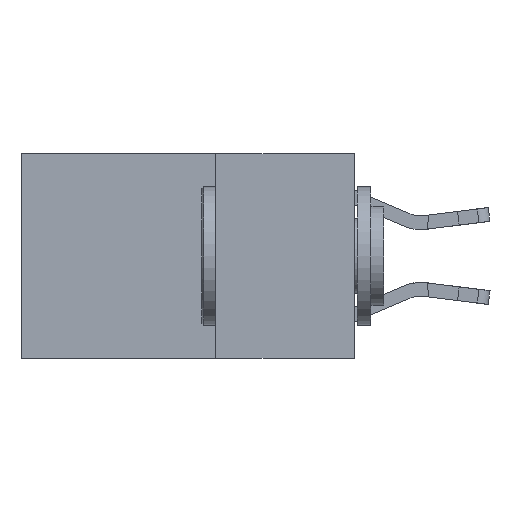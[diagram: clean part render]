
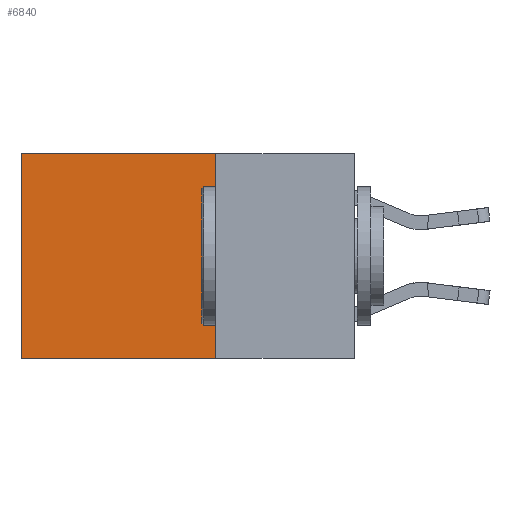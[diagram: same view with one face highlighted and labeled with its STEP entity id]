
A CAD part, left-side view. The second image highlights one B-rep face of the part: STEP entity #6840.
In plain terms, the highlighted planar face has unit normal (-1, 0, 0).
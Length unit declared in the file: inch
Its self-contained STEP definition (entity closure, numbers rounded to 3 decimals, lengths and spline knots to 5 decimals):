
#221 = EDGE_CURVE ( 'NONE', #16723, #18748, #11896, .T. ) ;
#668 = VERTEX_POINT ( 'NONE', #5026 ) ;
#800 = ORIENTED_EDGE ( 'NONE', *, *, #17229, .F. ) ;
#1386 = EDGE_CURVE ( 'NONE', #20524, #16723, #6756, .T. ) ;
#2444 = VECTOR ( 'NONE', #19869, 39.37008 ) ;
#2572 = CARTESIAN_POINT ( 'NONE',  ( 0.2625, 0.25, 0. ) ) ;
#2599 = VECTOR ( 'NONE', #14347, 39.37008 ) ;
#3278 = PLANE ( 'NONE',  #14975 ) ;
#4190 = ORIENTED_EDGE ( 'NONE', *, *, #1386, .T. ) ;
#4324 = CARTESIAN_POINT ( 'NONE',  ( 0.2625, 0.25, 0. ) ) ;
#4448 = FACE_OUTER_BOUND ( 'NONE', #17759, .T. ) ;
#4531 = CARTESIAN_POINT ( 'NONE',  ( 0.2625, 0.6, -0.37 ) ) ;
#5026 = CARTESIAN_POINT ( 'NONE',  ( 0.2625, 0.25, -0.37 ) ) ;
#5356 = CARTESIAN_POINT ( 'NONE',  ( 0.2625, 0.6, 0. ) ) ;
#6537 = CARTESIAN_POINT ( 'NONE',  ( 0.2625, 0.25, 0. ) ) ;
#6756 = LINE ( 'NONE', #6537, #2444 ) ;
#6840 = ADVANCED_FACE ( 'NONE', ( #4448 ), #3278, .F. ) ;
#7981 = DIRECTION ( 'NONE',  ( 0., 0., -1. ) ) ;
#9374 = DIRECTION ( 'NONE',  ( 1., 0., 0. ) ) ;
#9791 = CARTESIAN_POINT ( 'NONE',  ( 0.2625, 0.25, 0. ) ) ;
#9908 = CARTESIAN_POINT ( 'NONE',  ( 0.2625, 0.6, 0. ) ) ;
#11394 = EDGE_CURVE ( 'NONE', #668, #18748, #18039, .T. ) ;
#11896 = LINE ( 'NONE', #5356, #12572 ) ;
#12434 = LINE ( 'NONE', #2572, #17606 ) ;
#12572 = VECTOR ( 'NONE', #16470, 39.37008 ) ;
#14347 = DIRECTION ( 'NONE',  ( 0., 1., 0. ) ) ;
#14975 = AXIS2_PLACEMENT_3D ( 'NONE', #9791, #9374, #7981 ) ;
#15706 = DIRECTION ( 'NONE',  ( 0., 0., -1. ) ) ;
#16451 = CARTESIAN_POINT ( 'NONE',  ( 0.2625, 0.25, -0.37 ) ) ;
#16470 = DIRECTION ( 'NONE',  ( 0., 0., -1. ) ) ;
#16723 = VERTEX_POINT ( 'NONE', #9908 ) ;
#17229 = EDGE_CURVE ( 'NONE', #20524, #668, #12434, .T. ) ;
#17606 = VECTOR ( 'NONE', #15706, 39.37008 ) ;
#17759 = EDGE_LOOP ( 'NONE', ( #20206, #20894, #800, #4190 ) ) ;
#18039 = LINE ( 'NONE', #16451, #2599 ) ;
#18748 = VERTEX_POINT ( 'NONE', #4531 ) ;
#19869 = DIRECTION ( 'NONE',  ( 0., 1., 0. ) ) ;
#20206 = ORIENTED_EDGE ( 'NONE', *, *, #221, .T. ) ;
#20524 = VERTEX_POINT ( 'NONE', #4324 ) ;
#20894 = ORIENTED_EDGE ( 'NONE', *, *, #11394, .F. ) ;
